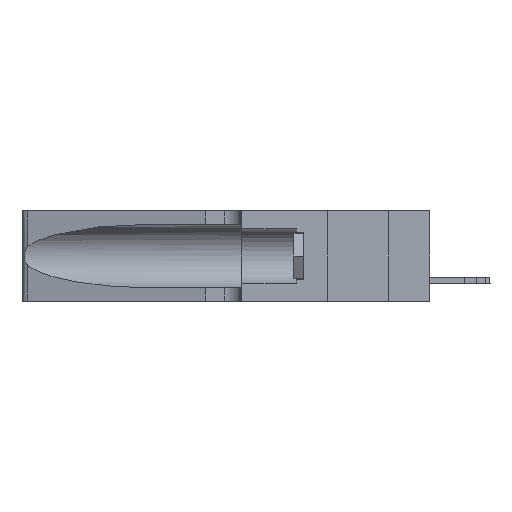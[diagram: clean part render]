
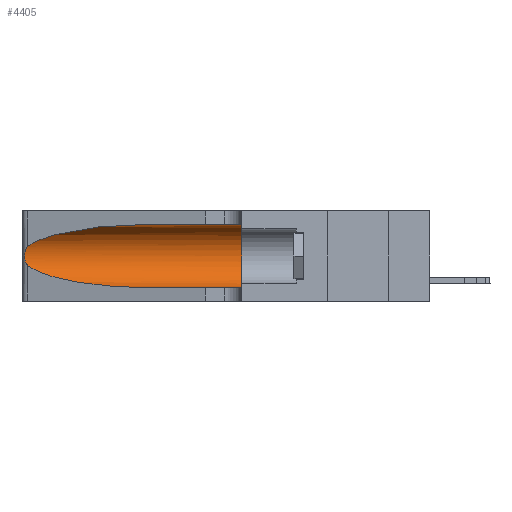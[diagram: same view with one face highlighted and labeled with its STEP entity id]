
A CAD part, left-side view. The second image highlights one B-rep face of the part: STEP entity #4405.
In plain terms, the highlighted cylindrical face has radius 3.308 mm (diameter 6.617 mm), a partial arc.
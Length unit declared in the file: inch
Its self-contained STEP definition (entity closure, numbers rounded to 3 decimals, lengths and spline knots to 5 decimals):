
#669 = VERTEX_POINT ( 'NONE', #14022 ) ;
#1366 = DIRECTION ( 'NONE',  ( 0., 1., 0. ) ) ;
#1546 = CARTESIAN_POINT ( 'NONE',  ( 0.25555, 1.22994, 0.2215 ) ) ;
#1581 = CARTESIAN_POINT ( 'NONE',  ( 0.25789, 1.23486, 0.15765 ) ) ;
#1801 = CARTESIAN_POINT ( 'NONE',  ( 0.26017, 1.23833, 0.17102 ) ) ;
#2757 = CARTESIAN_POINT ( 'NONE',  ( 0.2373, 1.15595, 0.28018 ) ) ;
#2849 = CARTESIAN_POINT ( 'NONE',  ( 0.1305, 0.35, 0.31525 ) ) ;
#2853 = B_SPLINE_CURVE_WITH_KNOTS ( 'NONE', 3,
 ( #14661, #1546, #14911, #22917, #33873, #10273, #18327, #14459, #1801, #15180, #1581, #28764, #29341, #7728 ),
 .UNSPECIFIED., .F., .F.,
 ( 4, 2, 2, 2, 2, 2, 4 ),
 ( 0., 0.00027, 0.00053, 0.00107, 0.0016, 0.00187, 0.00214 ),
 .UNSPECIFIED. ) ;
#2980 = VECTOR ( 'NONE', #29894, 39.37008 ) ;
#3484 = CARTESIAN_POINT ( 'NONE',  ( 0.25487, 1.22718, 0.14631 ) ) ;
#3876 = ORIENTED_EDGE ( 'NONE', *, *, #16468, .F. ) ;
#4405 = ADVANCED_FACE ( 'NONE', ( #22977 ), #8010, .F. ) ;
#5067 = LINE ( 'NONE', #21967, #2980 ) ;
#5330 = VERTEX_POINT ( 'NONE', #10325 ) ;
#6981 = ORIENTED_EDGE ( 'NONE', *, *, #23205, .T. ) ;
#7000 = CARTESIAN_POINT ( 'NONE',  ( 0.25487, 1.22718, 0.14631 ) ) ;
#7728 = CARTESIAN_POINT ( 'NONE',  ( 0.25487, 1.22718, 0.14631 ) ) ;
#8010 = CYLINDRICAL_SURFACE ( 'NONE', #20118, 0.13025 ) ;
#8653 = CARTESIAN_POINT ( 'NONE',  ( 0.25487, 1.22718, 0.22369 ) ) ;
#10273 = CARTESIAN_POINT ( 'NONE',  ( 0.26018, 1.23835, 0.19895 ) ) ;
#10325 = CARTESIAN_POINT ( 'NONE',  ( 0.25487, 1.22718, 0.22369 ) ) ;
#11237 = CARTESIAN_POINT ( 'NONE',  ( 0.18966, 0.96281, 0.31525 ) ) ;
#11606 = CARTESIAN_POINT ( 'NONE',  ( 0.1305, 0.72297, 0.05475 ) ) ;
#14022 = CARTESIAN_POINT ( 'NONE',  ( 0.1305, 0.35, 0.05475 ) ) ;
#14459 = CARTESIAN_POINT ( 'NONE',  ( 0.26075, 1.23896, 0.178 ) ) ;
#14549 = EDGE_CURVE ( 'NONE', #29529, #669, #33742, .T. ) ;
#14591 = EDGE_LOOP ( 'NONE', ( #30612, #6981, #33362, #31261, #3876, #24755 ) ) ;
#14661 = CARTESIAN_POINT ( 'NONE',  ( 0.25487, 1.22718, 0.22369 ) ) ;
#14911 = CARTESIAN_POINT ( 'NONE',  ( 0.25639, 1.23184, 0.21858 ) ) ;
#15180 = CARTESIAN_POINT ( 'NONE',  ( 0.25856, 1.23593, 0.16098 ) ) ;
#15877 = EDGE_CURVE ( 'NONE', #21558, #5330, #20547, .T. ) ;
#16468 = EDGE_CURVE ( 'NONE', #30602, #669, #31911, .T. ) ;
#16672 = DIRECTION ( 'NONE',  ( 0., 0., -1. ) ) ;
#17406 =( BOUNDED_CURVE ( )  B_SPLINE_CURVE ( 3, ( #3484, #24759, #27531, #11606 ),
 .UNSPECIFIED., .F., .F. ) 
 B_SPLINE_CURVE_WITH_KNOTS ( ( 4, 4 ),
 ( 3.44316, 4.71239 ),
 .UNSPECIFIED. ) 
 CURVE ( )  GEOMETRIC_REPRESENTATION_ITEM ( )  RATIONAL_B_SPLINE_CURVE ( ( 1., 0.87, 0.87, 1. ) ) 
 REPRESENTATION_ITEM ( '' )  );
#18327 = CARTESIAN_POINT ( 'NONE',  ( 0.26075, 1.23896, 0.19203 ) ) ;
#18982 = DIRECTION ( 'NONE',  ( 0., -1., 0. ) ) ;
#20118 = AXIS2_PLACEMENT_3D ( 'NONE', #23904, #26223, #16672 ) ;
#20547 =( BOUNDED_CURVE ( )  B_SPLINE_CURVE ( 3, ( #32182, #11237, #2757, #8653 ),
 .UNSPECIFIED., .F., .T. ) 
 B_SPLINE_CURVE_WITH_KNOTS ( ( 4, 4 ),
 ( 1.5708, 2.84003 ),
 .UNSPECIFIED. ) 
 CURVE ( )  GEOMETRIC_REPRESENTATION_ITEM ( )  RATIONAL_B_SPLINE_CURVE ( ( 1., 0.87, 0.87, 1. ) ) 
 REPRESENTATION_ITEM ( '' )  );
#20887 = EDGE_CURVE ( 'NONE', #24745, #29529, #17406, .T. ) ;
#21558 = VERTEX_POINT ( 'NONE', #29194 ) ;
#21967 = CARTESIAN_POINT ( 'NONE',  ( 0.1305, 1.61858, 0.31525 ) ) ;
#22123 = CARTESIAN_POINT ( 'NONE',  ( 0.1305, 0.72297, 0.05475 ) ) ;
#22917 = CARTESIAN_POINT ( 'NONE',  ( 0.25787, 1.23484, 0.2124 ) ) ;
#22977 = FACE_OUTER_BOUND ( 'NONE', #14591, .T. ) ;
#23205 = EDGE_CURVE ( 'NONE', #5330, #24745, #2853, .T. ) ;
#23904 = CARTESIAN_POINT ( 'NONE',  ( 0.1305, 1.61858, 0.185 ) ) ;
#24745 = VERTEX_POINT ( 'NONE', #7000 ) ;
#24755 = ORIENTED_EDGE ( 'NONE', *, *, #34094, .F. ) ;
#24759 = CARTESIAN_POINT ( 'NONE',  ( 0.2373, 1.15595, 0.08982 ) ) ;
#25310 = DIRECTION ( 'NONE',  ( 0., 0., 1. ) ) ;
#26223 = DIRECTION ( 'NONE',  ( 0., -1., 0. ) ) ;
#27531 = CARTESIAN_POINT ( 'NONE',  ( 0.18966, 0.96281, 0.05475 ) ) ;
#28764 = CARTESIAN_POINT ( 'NONE',  ( 0.25639, 1.23186, 0.15144 ) ) ;
#29194 = CARTESIAN_POINT ( 'NONE',  ( 0.1305, 0.72297, 0.31525 ) ) ;
#29326 = CARTESIAN_POINT ( 'NONE',  ( 0.1305, 1.61858, 0.05475 ) ) ;
#29341 = CARTESIAN_POINT ( 'NONE',  ( 0.25555, 1.22993, 0.14849 ) ) ;
#29529 = VERTEX_POINT ( 'NONE', #22123 ) ;
#29894 = DIRECTION ( 'NONE',  ( 0., -1., 0. ) ) ;
#29974 = VECTOR ( 'NONE', #18982, 39.37008 ) ;
#30602 = VERTEX_POINT ( 'NONE', #2849 ) ;
#30612 = ORIENTED_EDGE ( 'NONE', *, *, #15877, .T. ) ;
#31261 = ORIENTED_EDGE ( 'NONE', *, *, #14549, .T. ) ;
#31911 = CIRCLE ( 'NONE', #32358, 0.13025 ) ;
#32182 = CARTESIAN_POINT ( 'NONE',  ( 0.1305, 0.72297, 0.31525 ) ) ;
#32358 = AXIS2_PLACEMENT_3D ( 'NONE', #33338, #1366, #25310 ) ;
#33338 = CARTESIAN_POINT ( 'NONE',  ( 0.1305, 0.35, 0.185 ) ) ;
#33362 = ORIENTED_EDGE ( 'NONE', *, *, #20887, .T. ) ;
#33742 = LINE ( 'NONE', #29326, #29974 ) ;
#33873 = CARTESIAN_POINT ( 'NONE',  ( 0.25854, 1.2359, 0.20912 ) ) ;
#34094 = EDGE_CURVE ( 'NONE', #21558, #30602, #5067, .T. ) ;
